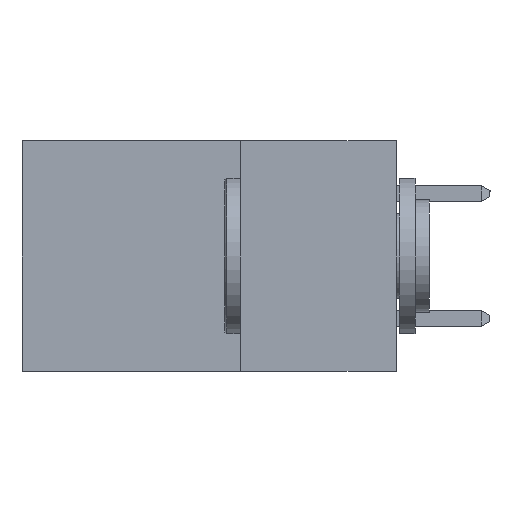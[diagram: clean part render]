
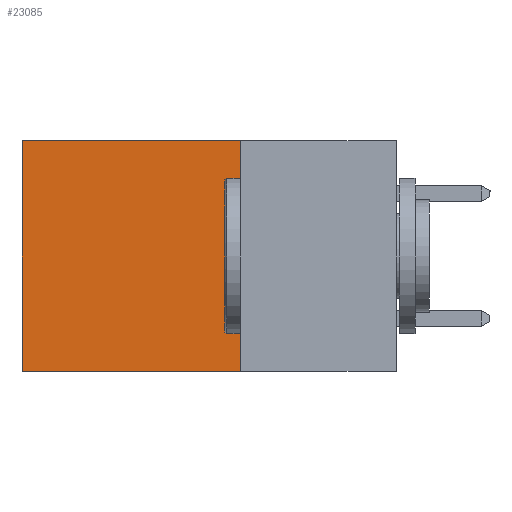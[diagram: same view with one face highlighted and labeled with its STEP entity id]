
A CAD part, left-side view. The second image highlights one B-rep face of the part: STEP entity #23085.
In plain terms, the highlighted planar face has unit normal (-1, 0, 0).
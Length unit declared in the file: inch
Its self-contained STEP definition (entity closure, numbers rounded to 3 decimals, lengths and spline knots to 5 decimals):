
#893 = CARTESIAN_POINT ( 'NONE',  ( 0.2615, 0.25, 0. ) ) ;
#1767 = ORIENTED_EDGE ( 'NONE', *, *, #12037, .T. ) ;
#3049 = DIRECTION ( 'NONE',  ( 0., 1., 0. ) ) ;
#3067 = LINE ( 'NONE', #26172, #15710 ) ;
#5191 = FACE_OUTER_BOUND ( 'NONE', #8152, .T. ) ;
#5582 = PLANE ( 'NONE',  #7646 ) ;
#6201 = EDGE_CURVE ( 'NONE', #7914, #11789, #16543, .T. ) ;
#7125 = CARTESIAN_POINT ( 'NONE',  ( 0.2615, 0.25, -0.37 ) ) ;
#7473 = DIRECTION ( 'NONE',  ( 0., 0., -1. ) ) ;
#7646 = AXIS2_PLACEMENT_3D ( 'NONE', #11672, #13558, #7473 ) ;
#7650 = DIRECTION ( 'NONE',  ( 0., 0., -1. ) ) ;
#7914 = VERTEX_POINT ( 'NONE', #7125 ) ;
#7935 = EDGE_CURVE ( 'NONE', #23710, #7914, #3067, .T. ) ;
#8152 = EDGE_LOOP ( 'NONE', ( #1767, #26601, #14164, #16295 ) ) ;
#8477 = CARTESIAN_POINT ( 'NONE',  ( 0.2615, 0.6, 0. ) ) ;
#8705 = CARTESIAN_POINT ( 'NONE',  ( 0.2615, 0.25, -0.37 ) ) ;
#11672 = CARTESIAN_POINT ( 'NONE',  ( 0.2615, 0.25, -0.37 ) ) ;
#11789 = VERTEX_POINT ( 'NONE', #13979 ) ;
#12037 = EDGE_CURVE ( 'NONE', #19328, #11789, #21395, .T. ) ;
#13558 = DIRECTION ( 'NONE',  ( 1., 0., 0. ) ) ;
#13979 = CARTESIAN_POINT ( 'NONE',  ( 0.2615, 0.6, -0.37 ) ) ;
#14164 = ORIENTED_EDGE ( 'NONE', *, *, #7935, .F. ) ;
#14566 = VECTOR ( 'NONE', #3049, 39.37008 ) ;
#14991 = VECTOR ( 'NONE', #25714, 39.37008 ) ;
#15098 = LINE ( 'NONE', #893, #14566 ) ;
#15710 = VECTOR ( 'NONE', #7650, 39.37008 ) ;
#16295 = ORIENTED_EDGE ( 'NONE', *, *, #20694, .T. ) ;
#16543 = LINE ( 'NONE', #8705, #19611 ) ;
#16950 = DIRECTION ( 'NONE',  ( 0., 1., 0. ) ) ;
#19328 = VERTEX_POINT ( 'NONE', #8477 ) ;
#19611 = VECTOR ( 'NONE', #16950, 39.37008 ) ;
#20694 = EDGE_CURVE ( 'NONE', #23710, #19328, #15098, .T. ) ;
#21130 = CARTESIAN_POINT ( 'NONE',  ( 0.2615, 0.6, -0.37 ) ) ;
#21395 = LINE ( 'NONE', #21130, #14991 ) ;
#23085 = ADVANCED_FACE ( 'NONE', ( #5191 ), #5582, .F. ) ;
#23710 = VERTEX_POINT ( 'NONE', #24210 ) ;
#24210 = CARTESIAN_POINT ( 'NONE',  ( 0.2615, 0.25, 0. ) ) ;
#25714 = DIRECTION ( 'NONE',  ( 0., 0., -1. ) ) ;
#26172 = CARTESIAN_POINT ( 'NONE',  ( 0.2615, 0.25, -0.37 ) ) ;
#26601 = ORIENTED_EDGE ( 'NONE', *, *, #6201, .F. ) ;
